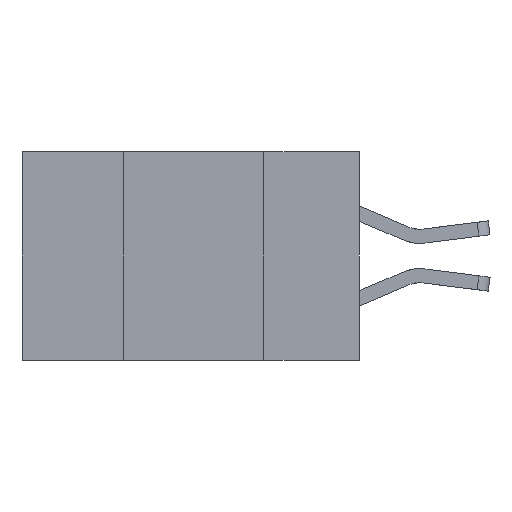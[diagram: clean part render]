
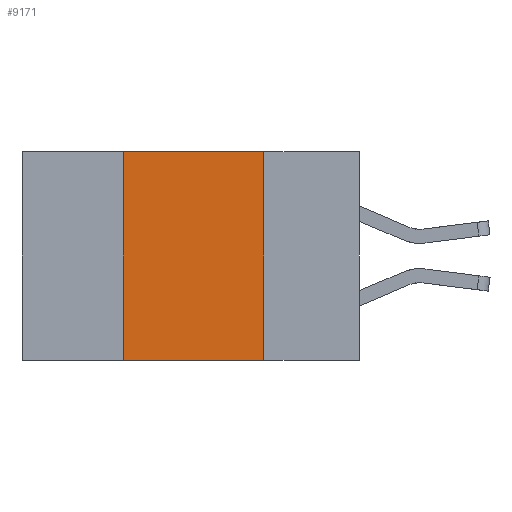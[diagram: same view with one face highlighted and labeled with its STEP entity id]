
A CAD part, left-side view. The second image highlights one B-rep face of the part: STEP entity #9171.
In plain terms, the highlighted planar face has unit normal (-1, 0, 0).
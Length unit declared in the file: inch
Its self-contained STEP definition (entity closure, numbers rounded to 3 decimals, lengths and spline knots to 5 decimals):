
#450 = CARTESIAN_POINT ( 'NONE',  ( 0., 0.17, -0.37 ) ) ;
#472 = VERTEX_POINT ( 'NONE', #2369 ) ;
#496 = VERTEX_POINT ( 'NONE', #6371 ) ;
#704 = DIRECTION ( 'NONE',  ( 0., 0., -1. ) ) ;
#1223 = CARTESIAN_POINT ( 'NONE',  ( 0., 0.42, 0. ) ) ;
#1475 = VECTOR ( 'NONE', #10423, 39.37008 ) ;
#1583 = FACE_OUTER_BOUND ( 'NONE', #7646, .T. ) ;
#1618 = DIRECTION ( 'NONE',  ( 0., -1., 0. ) ) ;
#2258 = CARTESIAN_POINT ( 'NONE',  ( 0., 0.6, 0. ) ) ;
#2331 = VECTOR ( 'NONE', #8520, 39.37008 ) ;
#2369 = CARTESIAN_POINT ( 'NONE',  ( 0., 0.42, -0.37 ) ) ;
#2408 = CARTESIAN_POINT ( 'NONE',  ( 0., 0.6, -0.37 ) ) ;
#2557 = LINE ( 'NONE', #1223, #2949 ) ;
#2680 = VECTOR ( 'NONE', #1618, 39.37008 ) ;
#2769 = VERTEX_POINT ( 'NONE', #450 ) ;
#2838 = LINE ( 'NONE', #2920, #2331 ) ;
#2920 = CARTESIAN_POINT ( 'NONE',  ( 0., 0.17, 0. ) ) ;
#2949 = VECTOR ( 'NONE', #3588, 39.37008 ) ;
#3588 = DIRECTION ( 'NONE',  ( 0., 0., 1. ) ) ;
#3817 = ORIENTED_EDGE ( 'NONE', *, *, #7334, .F. ) ;
#4273 = EDGE_CURVE ( 'NONE', #8975, #2769, #2838, .T. ) ;
#4701 = EDGE_CURVE ( 'NONE', #472, #496, #2557, .T. ) ;
#4920 = ORIENTED_EDGE ( 'NONE', *, *, #6145, .T. ) ;
#5269 = LINE ( 'NONE', #2258, #1475 ) ;
#5573 = CARTESIAN_POINT ( 'NONE',  ( 0., 0.6, 0. ) ) ;
#5835 = LINE ( 'NONE', #2408, #2680 ) ;
#6145 = EDGE_CURVE ( 'NONE', #472, #2769, #5835, .T. ) ;
#6371 = CARTESIAN_POINT ( 'NONE',  ( 0., 0.42, 0. ) ) ;
#7122 = ORIENTED_EDGE ( 'NONE', *, *, #4701, .F. ) ;
#7280 = DIRECTION ( 'NONE',  ( 1., 0., 0. ) ) ;
#7313 = AXIS2_PLACEMENT_3D ( 'NONE', #5573, #7280, #704 ) ;
#7334 = EDGE_CURVE ( 'NONE', #496, #8975, #5269, .T. ) ;
#7646 = EDGE_LOOP ( 'NONE', ( #8187, #3817, #7122, #4920 ) ) ;
#7705 = CARTESIAN_POINT ( 'NONE',  ( 0., 0.17, 0. ) ) ;
#8187 = ORIENTED_EDGE ( 'NONE', *, *, #4273, .F. ) ;
#8520 = DIRECTION ( 'NONE',  ( 0., 0., -1. ) ) ;
#8975 = VERTEX_POINT ( 'NONE', #7705 ) ;
#9171 = ADVANCED_FACE ( 'NONE', ( #1583 ), #9630, .F. ) ;
#9630 = PLANE ( 'NONE',  #7313 ) ;
#10423 = DIRECTION ( 'NONE',  ( 0., -1., 0. ) ) ;
